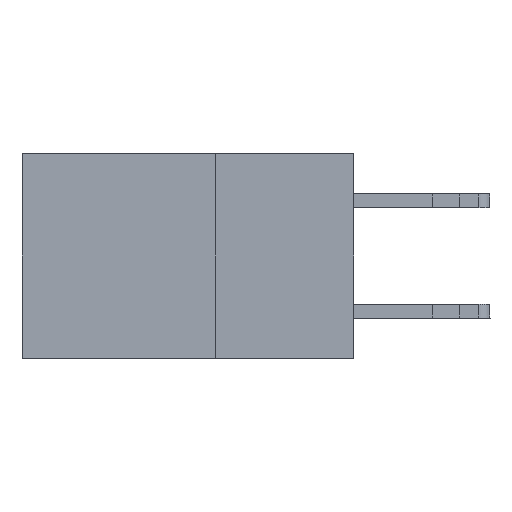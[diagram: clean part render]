
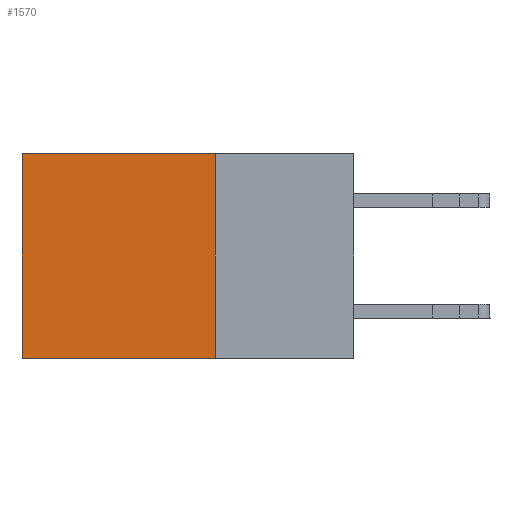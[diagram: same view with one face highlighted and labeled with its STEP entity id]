
A CAD part, left-side view. The second image highlights one B-rep face of the part: STEP entity #1570.
In plain terms, the highlighted planar face has unit normal (-1, 0, 0).
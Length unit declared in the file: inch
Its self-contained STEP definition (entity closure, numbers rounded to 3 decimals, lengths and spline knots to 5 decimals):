
#607 = VERTEX_POINT ( 'NONE', #7723 ) ;
#1570 = ADVANCED_FACE ( 'NONE', ( #16613 ), #8387, .F. ) ;
#3140 = DIRECTION ( 'NONE',  ( 0., 1., 0. ) ) ;
#4158 = ORIENTED_EDGE ( 'NONE', *, *, #9713, .F. ) ;
#4692 = EDGE_LOOP ( 'NONE', ( #9745, #9553, #4158, #15596 ) ) ;
#5013 = CARTESIAN_POINT ( 'NONE',  ( 0.2875, 0.25, 0. ) ) ;
#5638 = EDGE_CURVE ( 'NONE', #607, #6724, #7449, .T. ) ;
#5735 = DIRECTION ( 'NONE',  ( 0., 1., 0. ) ) ;
#6247 = LINE ( 'NONE', #14649, #10065 ) ;
#6724 = VERTEX_POINT ( 'NONE', #16322 ) ;
#7060 = CARTESIAN_POINT ( 'NONE',  ( 0.2875, 0.25, 0. ) ) ;
#7449 = LINE ( 'NONE', #16795, #14656 ) ;
#7480 = DIRECTION ( 'NONE',  ( 1., 0., 0. ) ) ;
#7723 = CARTESIAN_POINT ( 'NONE',  ( 0.2875, 0.6, 0. ) ) ;
#8387 = PLANE ( 'NONE',  #10893 ) ;
#8589 = EDGE_CURVE ( 'NONE', #15300, #607, #9515, .T. ) ;
#9515 = LINE ( 'NONE', #14342, #13794 ) ;
#9553 = ORIENTED_EDGE ( 'NONE', *, *, #12616, .F. ) ;
#9713 = EDGE_CURVE ( 'NONE', #15300, #10468, #17154, .T. ) ;
#9745 = ORIENTED_EDGE ( 'NONE', *, *, #5638, .T. ) ;
#10065 = VECTOR ( 'NONE', #3140, 39.37008 ) ;
#10468 = VERTEX_POINT ( 'NONE', #14220 ) ;
#10893 = AXIS2_PLACEMENT_3D ( 'NONE', #16527, #7480, #12827 ) ;
#12441 = DIRECTION ( 'NONE',  ( 0., 0., -1. ) ) ;
#12616 = EDGE_CURVE ( 'NONE', #10468, #6724, #6247, .T. ) ;
#12827 = DIRECTION ( 'NONE',  ( 0., 0., -1. ) ) ;
#13794 = VECTOR ( 'NONE', #5735, 39.37008 ) ;
#14220 = CARTESIAN_POINT ( 'NONE',  ( 0.2875, 0.25, -0.37 ) ) ;
#14342 = CARTESIAN_POINT ( 'NONE',  ( 0.2875, 0.25, 0. ) ) ;
#14649 = CARTESIAN_POINT ( 'NONE',  ( 0.2875, 0.25, -0.37 ) ) ;
#14656 = VECTOR ( 'NONE', #12441, 39.37008 ) ;
#15300 = VERTEX_POINT ( 'NONE', #5013 ) ;
#15596 = ORIENTED_EDGE ( 'NONE', *, *, #8589, .T. ) ;
#16322 = CARTESIAN_POINT ( 'NONE',  ( 0.2875, 0.6, -0.37 ) ) ;
#16527 = CARTESIAN_POINT ( 'NONE',  ( 0.2875, 0.25, 0. ) ) ;
#16613 = FACE_OUTER_BOUND ( 'NONE', #4692, .T. ) ;
#16795 = CARTESIAN_POINT ( 'NONE',  ( 0.2875, 0.6, 0. ) ) ;
#17125 = DIRECTION ( 'NONE',  ( 0., 0., -1. ) ) ;
#17154 = LINE ( 'NONE', #7060, #17585 ) ;
#17585 = VECTOR ( 'NONE', #17125, 39.37008 ) ;
